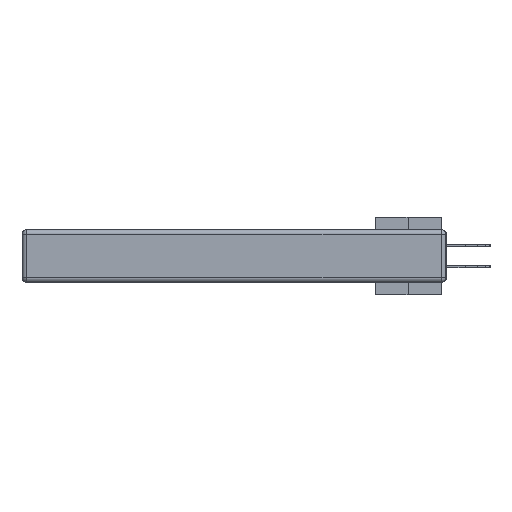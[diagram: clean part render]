
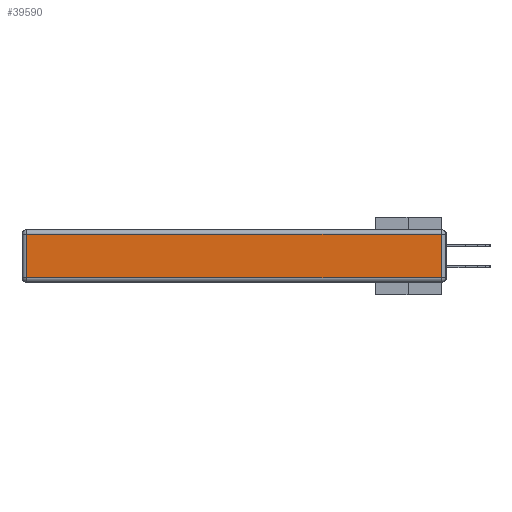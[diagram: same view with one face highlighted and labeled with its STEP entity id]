
A CAD part, left-side view. The second image highlights one B-rep face of the part: STEP entity #39590.
In plain terms, the highlighted planar face has unit normal (-1, 0, 0).
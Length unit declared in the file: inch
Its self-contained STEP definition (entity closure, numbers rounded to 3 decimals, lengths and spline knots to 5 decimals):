
#939 = VERTEX_POINT ( 'NONE', #15603 ) ;
#1462 = VERTEX_POINT ( 'NONE', #22220 ) ;
#1470 = DIRECTION ( 'NONE',  ( 0., 0., 1. ) ) ;
#2297 = FACE_OUTER_BOUND ( 'NONE', #30390, .T. ) ;
#2935 = CARTESIAN_POINT ( 'NONE',  ( 0., 0., -0.343 ) ) ;
#5704 = DIRECTION ( 'NONE',  ( 0., 1., 0. ) ) ;
#6673 = EDGE_CURVE ( 'NONE', #8922, #11211, #22022, .T. ) ;
#8922 = VERTEX_POINT ( 'NONE', #23546 ) ;
#10851 = EDGE_CURVE ( 'NONE', #11211, #939, #21391, .T. ) ;
#11211 = VERTEX_POINT ( 'NONE', #15525 ) ;
#11726 = EDGE_CURVE ( 'NONE', #939, #1462, #16805, .T. ) ;
#11866 = CARTESIAN_POINT ( 'NONE',  ( 0., 2.75, -0.03 ) ) ;
#12225 = DIRECTION ( 'NONE',  ( -1., 0., 0. ) ) ;
#12578 = AXIS2_PLACEMENT_3D ( 'NONE', #2935, #12225, #33269 ) ;
#14312 = ORIENTED_EDGE ( 'NONE', *, *, #11726, .T. ) ;
#15525 = CARTESIAN_POINT ( 'NONE',  ( 0., 2.72, -0.313 ) ) ;
#15603 = CARTESIAN_POINT ( 'NONE',  ( 0., 0.03, -0.313 ) ) ;
#15743 = CARTESIAN_POINT ( 'NONE',  ( 0., 2.72, -0.343 ) ) ;
#16805 = LINE ( 'NONE', #20211, #28213 ) ;
#17208 = ORIENTED_EDGE ( 'NONE', *, *, #20853, .T. ) ;
#20211 = CARTESIAN_POINT ( 'NONE',  ( 0., 0.03, -0.343 ) ) ;
#20443 = VECTOR ( 'NONE', #37709, 39.37008 ) ;
#20853 = EDGE_CURVE ( 'NONE', #1462, #8922, #35560, .T. ) ;
#21391 = LINE ( 'NONE', #33701, #20443 ) ;
#22022 = LINE ( 'NONE', #15743, #35372 ) ;
#22074 = DIRECTION ( 'NONE',  ( 0., 0., -1. ) ) ;
#22220 = CARTESIAN_POINT ( 'NONE',  ( 0., 0.03, -0.03 ) ) ;
#23546 = CARTESIAN_POINT ( 'NONE',  ( 0., 2.72, -0.03 ) ) ;
#25504 = VECTOR ( 'NONE', #5704, 39.37008 ) ;
#26823 = ORIENTED_EDGE ( 'NONE', *, *, #10851, .T. ) ;
#26976 = PLANE ( 'NONE',  #12578 ) ;
#28213 = VECTOR ( 'NONE', #1470, 39.37008 ) ;
#30390 = EDGE_LOOP ( 'NONE', ( #26823, #14312, #17208, #31673 ) ) ;
#31673 = ORIENTED_EDGE ( 'NONE', *, *, #6673, .T. ) ;
#33269 = DIRECTION ( 'NONE',  ( 0., 0., 1. ) ) ;
#33701 = CARTESIAN_POINT ( 'NONE',  ( 0., 0., -0.313 ) ) ;
#35372 = VECTOR ( 'NONE', #22074, 39.37008 ) ;
#35560 = LINE ( 'NONE', #11866, #25504 ) ;
#37709 = DIRECTION ( 'NONE',  ( 0., -1., 0. ) ) ;
#39590 = ADVANCED_FACE ( 'NONE', ( #2297 ), #26976, .T. ) ;
